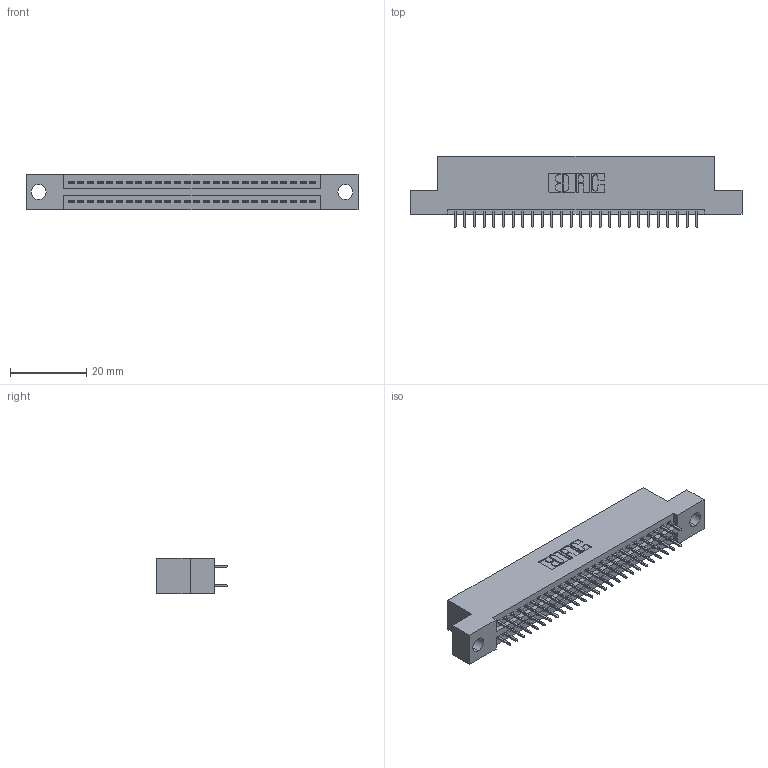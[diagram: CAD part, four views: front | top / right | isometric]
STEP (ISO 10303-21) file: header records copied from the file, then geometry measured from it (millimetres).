
FILE_DESCRIPTION (( 'STEP AP203' ), '1' );
FILE_NAME ('345-052-525-204.STEP', '2020-09-20T15:40:00', ( '' ), ( '' ), 'SwSTEP 2.0', 'SolidWorks 2020', '' );
FILE_SCHEMA (( 'CONFIG_CONTROL_DESIGN' ));
Length unit declared in the file: inch
Products named in the file (3): 345 Part_Flush Mounting Lugs - 0.156 Dia-TH; 345-292-001_345-293-125; 345-052-525-204
Assembly tree (53 placements, depth 2):
  345-052-525-204
    345 Part_Flush Mounting Lugs - 0.156 Dia-TH
    345-292-001_345-293-125  x52
Bounding box: 87.25 x 18.72 x 9.4 mm (x, y, z)
Volume: 8153.5 mm3; surface area: 11299.6 mm2
Topology: 53 solids, 53 shells, 2934 faces, 8297 edges, 5322 vertices
Faces by surface type: plane 2108, cylinder 826
Entity records: 22631 total; most frequent: CARTESIAN_POINT 3808, ORIENTED_EDGE 3742, DIRECTION 3379, EDGE_CURVE 1871, LINE 1639, VECTOR 1639, VERTEX_POINT 1242, AXIS2_PLACEMENT_3D 870
